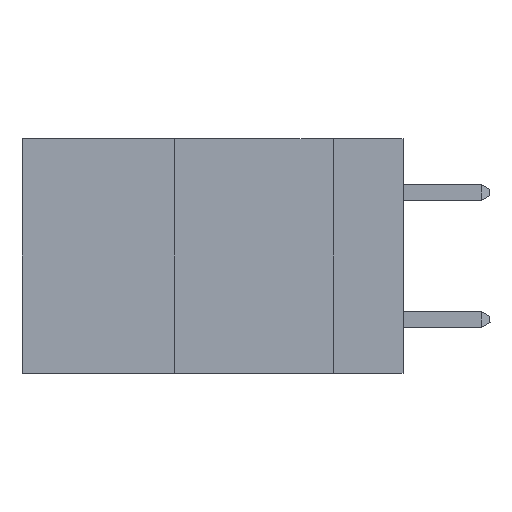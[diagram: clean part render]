
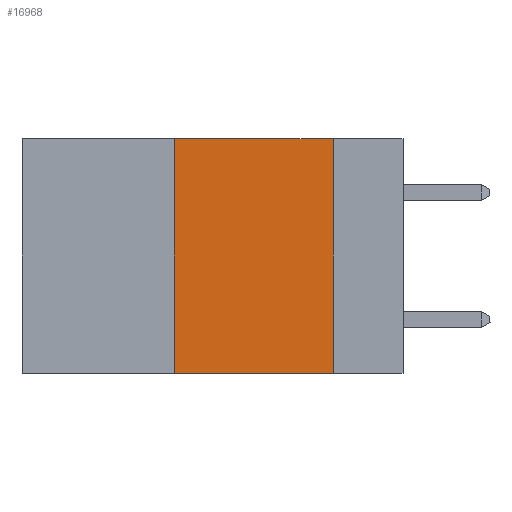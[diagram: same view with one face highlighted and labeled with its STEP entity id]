
A CAD part, left-side view. The second image highlights one B-rep face of the part: STEP entity #16968.
In plain terms, the highlighted planar face has unit normal (-1, 0, 0).
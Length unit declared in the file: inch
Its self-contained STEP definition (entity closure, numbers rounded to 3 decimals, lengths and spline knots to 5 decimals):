
#373 = ORIENTED_EDGE ( 'NONE', *, *, #3887, .F. ) ;
#1198 = DIRECTION ( 'NONE',  ( 0., 0., -1. ) ) ;
#2527 = EDGE_CURVE ( 'NONE', #10179, #8292, #5731, .T. ) ;
#2893 = CARTESIAN_POINT ( 'NONE',  ( 0., 0.11, 0. ) ) ;
#3056 = FACE_OUTER_BOUND ( 'NONE', #14973, .T. ) ;
#3887 = EDGE_CURVE ( 'NONE', #21543, #11606, #6973, .T. ) ;
#5731 = LINE ( 'NONE', #15229, #7235 ) ;
#5958 = DIRECTION ( 'NONE',  ( 0., -1., 0. ) ) ;
#6362 = DIRECTION ( 'NONE',  ( 0., 0., 1. ) ) ;
#6549 = DIRECTION ( 'NONE',  ( 1., 0., 0. ) ) ;
#6952 = VECTOR ( 'NONE', #1198, 39.37008 ) ;
#6973 = LINE ( 'NONE', #7086, #8371 ) ;
#7047 = EDGE_CURVE ( 'NONE', #11606, #8292, #23356, .T. ) ;
#7086 = CARTESIAN_POINT ( 'NONE',  ( 0., 0.6, 0. ) ) ;
#7235 = VECTOR ( 'NONE', #5958, 39.37008 ) ;
#7475 = LINE ( 'NONE', #22854, #19822 ) ;
#8292 = VERTEX_POINT ( 'NONE', #17011 ) ;
#8348 = CARTESIAN_POINT ( 'NONE',  ( 0., 0.6, 0. ) ) ;
#8371 = VECTOR ( 'NONE', #9020, 39.37008 ) ;
#9020 = DIRECTION ( 'NONE',  ( 0., -1., 0. ) ) ;
#10179 = VERTEX_POINT ( 'NONE', #15448 ) ;
#10399 = PLANE ( 'NONE',  #20107 ) ;
#11606 = VERTEX_POINT ( 'NONE', #12657 ) ;
#11820 = ORIENTED_EDGE ( 'NONE', *, *, #2527, .T. ) ;
#12657 = CARTESIAN_POINT ( 'NONE',  ( 0., 0.11, 0. ) ) ;
#14642 = EDGE_CURVE ( 'NONE', #10179, #21543, #7475, .T. ) ;
#14973 = EDGE_LOOP ( 'NONE', ( #20754, #373, #18031, #11820 ) ) ;
#15229 = CARTESIAN_POINT ( 'NONE',  ( 0., 0.6, -0.37 ) ) ;
#15448 = CARTESIAN_POINT ( 'NONE',  ( 0., 0.36, -0.37 ) ) ;
#16968 = ADVANCED_FACE ( 'NONE', ( #3056 ), #10399, .F. ) ;
#17011 = CARTESIAN_POINT ( 'NONE',  ( 0., 0.11, -0.37 ) ) ;
#17744 = DIRECTION ( 'NONE',  ( 0., 0., -1. ) ) ;
#18031 = ORIENTED_EDGE ( 'NONE', *, *, #14642, .F. ) ;
#19822 = VECTOR ( 'NONE', #6362, 39.37008 ) ;
#19958 = CARTESIAN_POINT ( 'NONE',  ( 0., 0.36, 0. ) ) ;
#20107 = AXIS2_PLACEMENT_3D ( 'NONE', #8348, #6549, #17744 ) ;
#20754 = ORIENTED_EDGE ( 'NONE', *, *, #7047, .F. ) ;
#21543 = VERTEX_POINT ( 'NONE', #19958 ) ;
#22854 = CARTESIAN_POINT ( 'NONE',  ( 0., 0.36, 0. ) ) ;
#23356 = LINE ( 'NONE', #2893, #6952 ) ;
